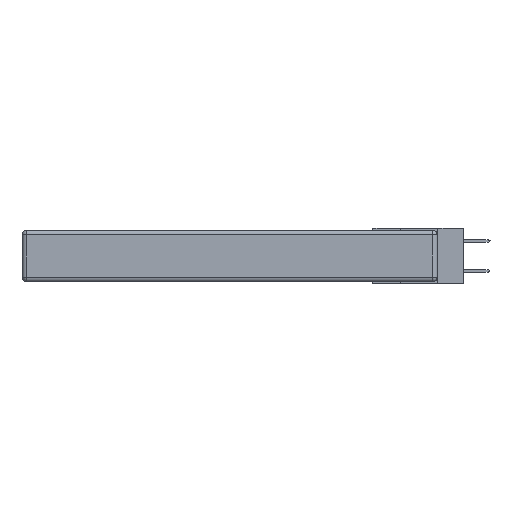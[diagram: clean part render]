
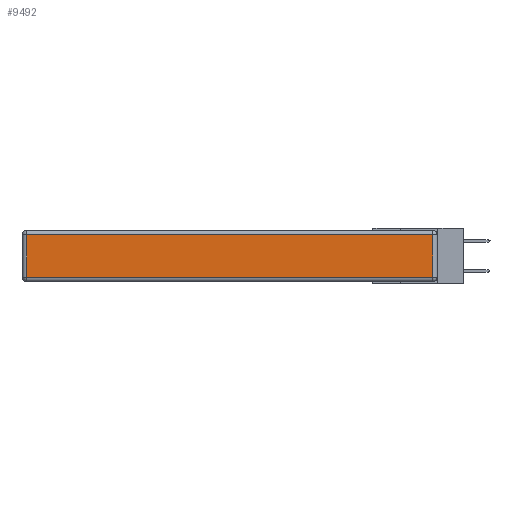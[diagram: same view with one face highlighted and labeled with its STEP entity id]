
A CAD part, left-side view. The second image highlights one B-rep face of the part: STEP entity #9492.
In plain terms, the highlighted planar face has unit normal (-1, 0, 0).
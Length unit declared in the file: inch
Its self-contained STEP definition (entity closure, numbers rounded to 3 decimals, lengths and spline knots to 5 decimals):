
#1020 = DIRECTION ( 'NONE',  ( 0., 0., 1. ) ) ;
#1361 = AXIS2_PLACEMENT_3D ( 'NONE', #17215, #10350, #1020 ) ;
#1758 = LINE ( 'NONE', #20750, #5386 ) ;
#1927 = ORIENTED_EDGE ( 'NONE', *, *, #11088, .T. ) ;
#2740 = ORIENTED_EDGE ( 'NONE', *, *, #14500, .T. ) ;
#4100 = CARTESIAN_POINT ( 'NONE',  ( 0., 2.72, -0.313 ) ) ;
#4378 = DIRECTION ( 'NONE',  ( 0., 1., 0. ) ) ;
#4599 = VECTOR ( 'NONE', #28037, 39.37008 ) ;
#4629 = CARTESIAN_POINT ( 'NONE',  ( 0., 2.72, -0.03 ) ) ;
#5386 = VECTOR ( 'NONE', #7209, 39.37008 ) ;
#5828 = VERTEX_POINT ( 'NONE', #4100 ) ;
#7209 = DIRECTION ( 'NONE',  ( 0., 0., -1. ) ) ;
#9492 = ADVANCED_FACE ( 'NONE', ( #20383 ), #21922, .T. ) ;
#9673 = VECTOR ( 'NONE', #4378, 39.37008 ) ;
#10350 = DIRECTION ( 'NONE',  ( -1., 0., 0. ) ) ;
#10688 = LINE ( 'NONE', #27830, #4599 ) ;
#10850 = ORIENTED_EDGE ( 'NONE', *, *, #13770, .T. ) ;
#11087 = CARTESIAN_POINT ( 'NONE',  ( 0., 2.75, -0.03 ) ) ;
#11088 = EDGE_CURVE ( 'NONE', #16572, #16346, #28562, .T. ) ;
#13768 = CARTESIAN_POINT ( 'NONE',  ( 0., 0.03, -0.313 ) ) ;
#13770 = EDGE_CURVE ( 'NONE', #29512, #5828, #1758, .T. ) ;
#14500 = EDGE_CURVE ( 'NONE', #16346, #29512, #18643, .T. ) ;
#16346 = VERTEX_POINT ( 'NONE', #28073 ) ;
#16572 = VERTEX_POINT ( 'NONE', #13768 ) ;
#17132 = CARTESIAN_POINT ( 'NONE',  ( 0., 0.03, -0.343 ) ) ;
#17215 = CARTESIAN_POINT ( 'NONE',  ( 0., 0., -0.343 ) ) ;
#18643 = LINE ( 'NONE', #11087, #9673 ) ;
#19934 = VECTOR ( 'NONE', #28852, 39.37008 ) ;
#20383 = FACE_OUTER_BOUND ( 'NONE', #22607, .T. ) ;
#20750 = CARTESIAN_POINT ( 'NONE',  ( 0., 2.72, -0.343 ) ) ;
#21922 = PLANE ( 'NONE',  #1361 ) ;
#22607 = EDGE_LOOP ( 'NONE', ( #22724, #1927, #2740, #10850 ) ) ;
#22724 = ORIENTED_EDGE ( 'NONE', *, *, #26456, .T. ) ;
#26456 = EDGE_CURVE ( 'NONE', #5828, #16572, #10688, .T. ) ;
#27830 = CARTESIAN_POINT ( 'NONE',  ( 0., 0., -0.313 ) ) ;
#28037 = DIRECTION ( 'NONE',  ( 0., -1., 0. ) ) ;
#28073 = CARTESIAN_POINT ( 'NONE',  ( 0., 0.03, -0.03 ) ) ;
#28562 = LINE ( 'NONE', #17132, #19934 ) ;
#28852 = DIRECTION ( 'NONE',  ( 0., 0., 1. ) ) ;
#29512 = VERTEX_POINT ( 'NONE', #4629 ) ;
